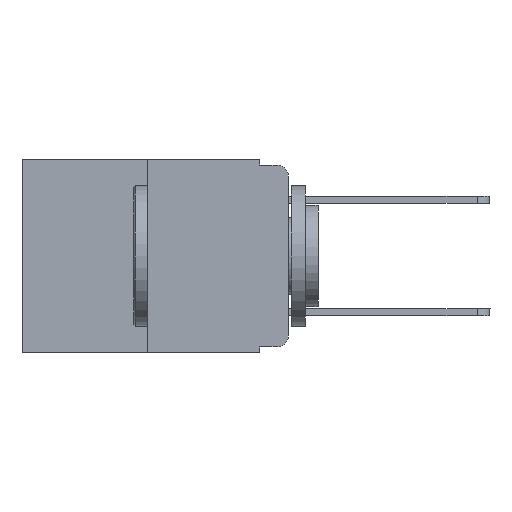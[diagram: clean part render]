
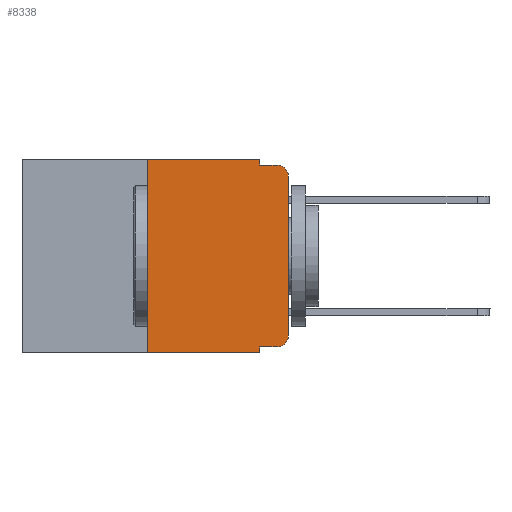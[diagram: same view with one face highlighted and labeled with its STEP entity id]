
A CAD part, left-side view. The second image highlights one B-rep face of the part: STEP entity #8338.
In plain terms, the highlighted planar face has unit normal (-1, 0, 0).
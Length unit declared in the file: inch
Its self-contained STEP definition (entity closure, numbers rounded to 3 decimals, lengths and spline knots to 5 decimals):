
#22 = EDGE_CURVE ( 'NONE', #7736, #22145, #2882, .T. ) ;
#426 = ORIENTED_EDGE ( 'NONE', *, *, #11469, .T. ) ;
#1742 = ORIENTED_EDGE ( 'NONE', *, *, #10578, .F. ) ;
#2283 = DIRECTION ( 'NONE',  ( 0., 0., -1. ) ) ;
#2816 = CARTESIAN_POINT ( 'NONE',  ( 0., 0.051, 0. ) ) ;
#2832 = CARTESIAN_POINT ( 'NONE',  ( 0., 0.051, -0.333 ) ) ;
#2882 = LINE ( 'NONE', #14415, #21304 ) ;
#3029 = CARTESIAN_POINT ( 'NONE',  ( 0., 0.051, 0. ) ) ;
#3476 = DIRECTION ( 'NONE',  ( 0., 0., -1. ) ) ;
#3924 = ORIENTED_EDGE ( 'NONE', *, *, #21460, .F. ) ;
#4631 = DIRECTION ( 'NONE',  ( 0., -1., 0. ) ) ;
#5059 = VECTOR ( 'NONE', #4631, 39.37008 ) ;
#5184 = EDGE_CURVE ( 'NONE', #8664, #12389, #16662, .T. ) ;
#5188 = VERTEX_POINT ( 'NONE', #15334 ) ;
#5344 = CARTESIAN_POINT ( 'NONE',  ( 0., 0.051, -0.333 ) ) ;
#5404 = DIRECTION ( 'NONE',  ( 0., -1., 0. ) ) ;
#5534 = VECTOR ( 'NONE', #14822, 39.37008 ) ;
#5725 = ORIENTED_EDGE ( 'NONE', *, *, #14914, .F. ) ;
#5777 = CIRCLE ( 'NONE', #20234, 0.02 ) ;
#5880 = CARTESIAN_POINT ( 'NONE',  ( 0., 0.051, 0. ) ) ;
#6210 = CARTESIAN_POINT ( 'NONE',  ( 0., 0.02, -0.03 ) ) ;
#6212 = LINE ( 'NONE', #3029, #15116 ) ;
#6579 = CIRCLE ( 'NONE', #21726, 0.02 ) ;
#6760 = CARTESIAN_POINT ( 'NONE',  ( 0., 0.051, -0.343 ) ) ;
#6874 = DIRECTION ( 'NONE',  ( 0., 0., -1. ) ) ;
#7353 = FACE_OUTER_BOUND ( 'NONE', #13472, .T. ) ;
#7494 = DIRECTION ( 'NONE',  ( 1., 0., 0. ) ) ;
#7736 = VERTEX_POINT ( 'NONE', #21916 ) ;
#7835 = DIRECTION ( 'NONE',  ( 0., 0., -1. ) ) ;
#7944 = CARTESIAN_POINT ( 'NONE',  ( 0., 0.02, -0.01 ) ) ;
#8285 = ORIENTED_EDGE ( 'NONE', *, *, #18318, .F. ) ;
#8338 = ADVANCED_FACE ( 'NONE', ( #7353 ), #18188, .F. ) ;
#8556 = DIRECTION ( 'NONE',  ( -1., 0., 0. ) ) ;
#8664 = VERTEX_POINT ( 'NONE', #19408 ) ;
#8935 = VECTOR ( 'NONE', #22464, 39.37008 ) ;
#9096 = CARTESIAN_POINT ( 'NONE',  ( 0., 0.25, 0. ) ) ;
#9622 = CARTESIAN_POINT ( 'NONE',  ( 0., 0.473, 0. ) ) ;
#9727 = DIRECTION ( 'NONE',  ( -1., 0., 0. ) ) ;
#9814 = VECTOR ( 'NONE', #21544, 39.37008 ) ;
#9887 = CARTESIAN_POINT ( 'NONE',  ( 0., 0.02, -0.333 ) ) ;
#10034 = EDGE_CURVE ( 'NONE', #11561, #14690, #15583, .T. ) ;
#10578 = EDGE_CURVE ( 'NONE', #5188, #19613, #15820, .T. ) ;
#11469 = EDGE_CURVE ( 'NONE', #12688, #8664, #5777, .T. ) ;
#11561 = VERTEX_POINT ( 'NONE', #15786 ) ;
#11795 = ORIENTED_EDGE ( 'NONE', *, *, #22, .F. ) ;
#11905 = ORIENTED_EDGE ( 'NONE', *, *, #5184, .T. ) ;
#12389 = VERTEX_POINT ( 'NONE', #19330 ) ;
#12688 = VERTEX_POINT ( 'NONE', #9887 ) ;
#12719 = EDGE_CURVE ( 'NONE', #12389, #22145, #6579, .T. ) ;
#13472 = EDGE_LOOP ( 'NONE', ( #11905, #17232, #11795, #8285, #1742, #5725, #16241, #3924, #15803, #426 ) ) ;
#14238 = LINE ( 'NONE', #2832, #5059 ) ;
#14415 = CARTESIAN_POINT ( 'NONE',  ( 0., 0.051, -0.01 ) ) ;
#14572 = CARTESIAN_POINT ( 'NONE',  ( 0., 0.473, 0. ) ) ;
#14623 = EDGE_CURVE ( 'NONE', #19734, #12688, #14238, .T. ) ;
#14690 = VERTEX_POINT ( 'NONE', #6760 ) ;
#14822 = DIRECTION ( 'NONE',  ( 0., -1., 0. ) ) ;
#14914 = EDGE_CURVE ( 'NONE', #11561, #5188, #16492, .T. ) ;
#15116 = VECTOR ( 'NONE', #6874, 39.37008 ) ;
#15286 = CARTESIAN_POINT ( 'NONE',  ( 0., 0.473, -0.343 ) ) ;
#15334 = CARTESIAN_POINT ( 'NONE',  ( 0., 0.25, 0. ) ) ;
#15442 = CARTESIAN_POINT ( 'NONE',  ( 0., 0., 0. ) ) ;
#15583 = LINE ( 'NONE', #15286, #8935 ) ;
#15786 = CARTESIAN_POINT ( 'NONE',  ( 0., 0.25, -0.343 ) ) ;
#15803 = ORIENTED_EDGE ( 'NONE', *, *, #14623, .T. ) ;
#15809 = AXIS2_PLACEMENT_3D ( 'NONE', #14572, #7494, #18041 ) ;
#15820 = LINE ( 'NONE', #9622, #5534 ) ;
#16241 = ORIENTED_EDGE ( 'NONE', *, *, #10034, .T. ) ;
#16492 = LINE ( 'NONE', #9096, #9814 ) ;
#16633 = VECTOR ( 'NONE', #2283, 39.37008 ) ;
#16662 = LINE ( 'NONE', #15442, #22498 ) ;
#17232 = ORIENTED_EDGE ( 'NONE', *, *, #12719, .T. ) ;
#17470 = LINE ( 'NONE', #5880, #16633 ) ;
#18041 = DIRECTION ( 'NONE',  ( 0., 0., -1. ) ) ;
#18188 = PLANE ( 'NONE',  #15809 ) ;
#18318 = EDGE_CURVE ( 'NONE', #19613, #7736, #6212, .T. ) ;
#19330 = CARTESIAN_POINT ( 'NONE',  ( 0., 0., -0.03 ) ) ;
#19408 = CARTESIAN_POINT ( 'NONE',  ( 0., 0., -0.313 ) ) ;
#19613 = VERTEX_POINT ( 'NONE', #2816 ) ;
#19734 = VERTEX_POINT ( 'NONE', #5344 ) ;
#20234 = AXIS2_PLACEMENT_3D ( 'NONE', #23033, #8556, #3476 ) ;
#21304 = VECTOR ( 'NONE', #5404, 39.37008 ) ;
#21460 = EDGE_CURVE ( 'NONE', #19734, #14690, #17470, .T. ) ;
#21544 = DIRECTION ( 'NONE',  ( 0., 0., 1. ) ) ;
#21651 = DIRECTION ( 'NONE',  ( 0., 0., 1. ) ) ;
#21726 = AXIS2_PLACEMENT_3D ( 'NONE', #6210, #9727, #7835 ) ;
#21916 = CARTESIAN_POINT ( 'NONE',  ( 0., 0.051, -0.01 ) ) ;
#22145 = VERTEX_POINT ( 'NONE', #7944 ) ;
#22464 = DIRECTION ( 'NONE',  ( 0., -1., 0. ) ) ;
#22498 = VECTOR ( 'NONE', #21651, 39.37008 ) ;
#23033 = CARTESIAN_POINT ( 'NONE',  ( 0., 0.02, -0.313 ) ) ;
